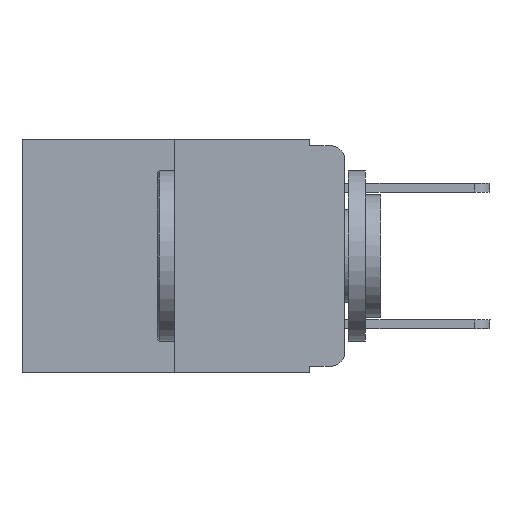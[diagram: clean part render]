
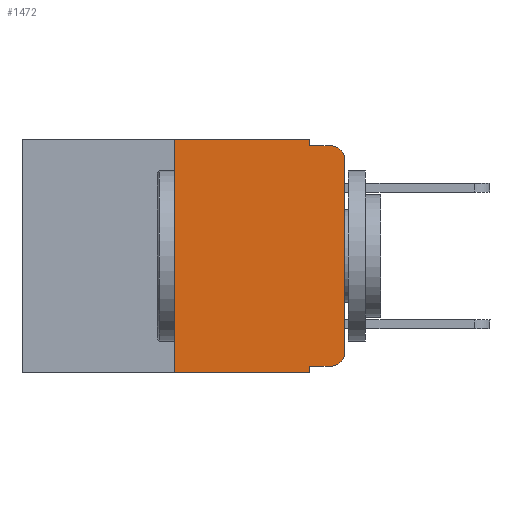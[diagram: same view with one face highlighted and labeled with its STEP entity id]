
A CAD part, left-side view. The second image highlights one B-rep face of the part: STEP entity #1472.
In plain terms, the highlighted planar face has unit normal (-1, 0, 0).
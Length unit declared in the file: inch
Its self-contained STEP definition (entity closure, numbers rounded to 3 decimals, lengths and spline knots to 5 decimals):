
#92 = FACE_OUTER_BOUND ( 'NONE', #3858, .T. ) ;
#539 = LINE ( 'NONE', #16305, #12967 ) ;
#797 = VERTEX_POINT ( 'NONE', #1685 ) ;
#972 = DIRECTION ( 'NONE',  ( 0., -1., 0. ) ) ;
#1054 = CARTESIAN_POINT ( 'NONE',  ( 0., 0.25, -0.343 ) ) ;
#1195 = LINE ( 'NONE', #6496, #13992 ) ;
#1220 = DIRECTION ( 'NONE',  ( 0., 0., -1. ) ) ;
#1334 = AXIS2_PLACEMENT_3D ( 'NONE', #14161, #5328, #1220 ) ;
#1418 = CARTESIAN_POINT ( 'NONE',  ( 0., 0.25, 0. ) ) ;
#1425 = VERTEX_POINT ( 'NONE', #11858 ) ;
#1437 = LINE ( 'NONE', #9424, #16953 ) ;
#1472 = ADVANCED_FACE ( 'NONE', ( #92 ), #10491, .F. ) ;
#1685 = CARTESIAN_POINT ( 'NONE',  ( 0., 0.051, 0. ) ) ;
#1692 = DIRECTION ( 'NONE',  ( 0., -1., 0. ) ) ;
#1761 = CARTESIAN_POINT ( 'NONE',  ( 0., 0.473, 0. ) ) ;
#1811 = ORIENTED_EDGE ( 'NONE', *, *, #9873, .F. ) ;
#2193 = VECTOR ( 'NONE', #13238, 39.37008 ) ;
#2229 = AXIS2_PLACEMENT_3D ( 'NONE', #9049, #14268, #8463 ) ;
#2328 = EDGE_CURVE ( 'NONE', #5179, #797, #12306, .T. ) ;
#2406 = CARTESIAN_POINT ( 'NONE',  ( 0., 0.02, -0.313 ) ) ;
#2923 = CARTESIAN_POINT ( 'NONE',  ( 0., 0., -0.03 ) ) ;
#3143 = EDGE_CURVE ( 'NONE', #5114, #7500, #13049, .T. ) ;
#3190 = DIRECTION ( 'NONE',  ( 0., -1., 0. ) ) ;
#3448 = CARTESIAN_POINT ( 'NONE',  ( 0., 0., -0.313 ) ) ;
#3858 = EDGE_LOOP ( 'NONE', ( #10292, #8489, #7033, #1811, #15765, #16073, #16864, #4972, #7163, #16248 ) ) ;
#4073 = VERTEX_POINT ( 'NONE', #2923 ) ;
#4182 = EDGE_CURVE ( 'NONE', #1425, #16497, #8335, .T. ) ;
#4573 = CARTESIAN_POINT ( 'NONE',  ( 0., 0.051, -0.01 ) ) ;
#4828 = CARTESIAN_POINT ( 'NONE',  ( 0., 0.051, -0.333 ) ) ;
#4972 = ORIENTED_EDGE ( 'NONE', *, *, #4182, .F. ) ;
#5114 = VERTEX_POINT ( 'NONE', #7080 ) ;
#5170 = CARTESIAN_POINT ( 'NONE',  ( 0., 0.051, -0.01 ) ) ;
#5179 = VERTEX_POINT ( 'NONE', #13856 ) ;
#5183 = VECTOR ( 'NONE', #8105, 39.37008 ) ;
#5328 = DIRECTION ( 'NONE',  ( 1., 0., 0. ) ) ;
#5353 = VECTOR ( 'NONE', #3190, 39.37008 ) ;
#6109 = LINE ( 'NONE', #4828, #15016 ) ;
#6496 = CARTESIAN_POINT ( 'NONE',  ( 0., 0.051, 0. ) ) ;
#6773 = EDGE_CURVE ( 'NONE', #7593, #16497, #1437, .T. ) ;
#6789 = LINE ( 'NONE', #5170, #2193 ) ;
#7033 = ORIENTED_EDGE ( 'NONE', *, *, #8959, .F. ) ;
#7080 = CARTESIAN_POINT ( 'NONE',  ( 0., 0.02, -0.333 ) ) ;
#7163 = ORIENTED_EDGE ( 'NONE', *, *, #7563, .T. ) ;
#7284 = AXIS2_PLACEMENT_3D ( 'NONE', #2406, #9185, #8935 ) ;
#7500 = VERTEX_POINT ( 'NONE', #3448 ) ;
#7563 = EDGE_CURVE ( 'NONE', #1425, #5114, #6109, .T. ) ;
#7583 = VECTOR ( 'NONE', #10995, 39.37008 ) ;
#7593 = VERTEX_POINT ( 'NONE', #1054 ) ;
#7926 = LINE ( 'NONE', #1418, #5183 ) ;
#8105 = DIRECTION ( 'NONE',  ( 0., 0., 1. ) ) ;
#8335 = LINE ( 'NONE', #13562, #7583 ) ;
#8336 = CARTESIAN_POINT ( 'NONE',  ( 0., 0.051, -0.343 ) ) ;
#8463 = DIRECTION ( 'NONE',  ( 0., 0., -1. ) ) ;
#8489 = ORIENTED_EDGE ( 'NONE', *, *, #10236, .T. ) ;
#8547 = EDGE_CURVE ( 'NONE', #7593, #5179, #7926, .T. ) ;
#8935 = DIRECTION ( 'NONE',  ( 0., 0., -1. ) ) ;
#8959 = EDGE_CURVE ( 'NONE', #16319, #15808, #6789, .T. ) ;
#9049 = CARTESIAN_POINT ( 'NONE',  ( 0., 0.02, -0.03 ) ) ;
#9185 = DIRECTION ( 'NONE',  ( -1., 0., 0. ) ) ;
#9424 = CARTESIAN_POINT ( 'NONE',  ( 0., 0.473, -0.343 ) ) ;
#9859 = CARTESIAN_POINT ( 'NONE',  ( 0., 0.02, -0.01 ) ) ;
#9873 = EDGE_CURVE ( 'NONE', #797, #16319, #1195, .T. ) ;
#10236 = EDGE_CURVE ( 'NONE', #4073, #15808, #13184, .T. ) ;
#10292 = ORIENTED_EDGE ( 'NONE', *, *, #14079, .T. ) ;
#10491 = PLANE ( 'NONE',  #1334 ) ;
#10995 = DIRECTION ( 'NONE',  ( 0., 0., -1. ) ) ;
#11858 = CARTESIAN_POINT ( 'NONE',  ( 0., 0.051, -0.333 ) ) ;
#12306 = LINE ( 'NONE', #1761, #5353 ) ;
#12558 = DIRECTION ( 'NONE',  ( 0., 0., 1. ) ) ;
#12959 = DIRECTION ( 'NONE',  ( 0., 0., -1. ) ) ;
#12967 = VECTOR ( 'NONE', #12558, 39.37008 ) ;
#13049 = CIRCLE ( 'NONE', #7284, 0.02 ) ;
#13184 = CIRCLE ( 'NONE', #2229, 0.02 ) ;
#13238 = DIRECTION ( 'NONE',  ( 0., -1., 0. ) ) ;
#13562 = CARTESIAN_POINT ( 'NONE',  ( 0., 0.051, 0. ) ) ;
#13856 = CARTESIAN_POINT ( 'NONE',  ( 0., 0.25, 0. ) ) ;
#13992 = VECTOR ( 'NONE', #12959, 39.37008 ) ;
#14079 = EDGE_CURVE ( 'NONE', #7500, #4073, #539, .T. ) ;
#14161 = CARTESIAN_POINT ( 'NONE',  ( 0., 0.473, 0. ) ) ;
#14268 = DIRECTION ( 'NONE',  ( -1., 0., 0. ) ) ;
#15016 = VECTOR ( 'NONE', #972, 39.37008 ) ;
#15765 = ORIENTED_EDGE ( 'NONE', *, *, #2328, .F. ) ;
#15808 = VERTEX_POINT ( 'NONE', #9859 ) ;
#16073 = ORIENTED_EDGE ( 'NONE', *, *, #8547, .F. ) ;
#16248 = ORIENTED_EDGE ( 'NONE', *, *, #3143, .T. ) ;
#16305 = CARTESIAN_POINT ( 'NONE',  ( 0., 0., 0. ) ) ;
#16319 = VERTEX_POINT ( 'NONE', #4573 ) ;
#16497 = VERTEX_POINT ( 'NONE', #8336 ) ;
#16864 = ORIENTED_EDGE ( 'NONE', *, *, #6773, .T. ) ;
#16953 = VECTOR ( 'NONE', #1692, 39.37008 ) ;
